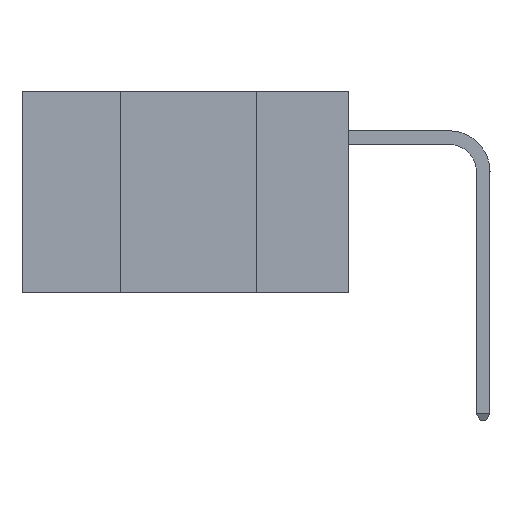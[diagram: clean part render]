
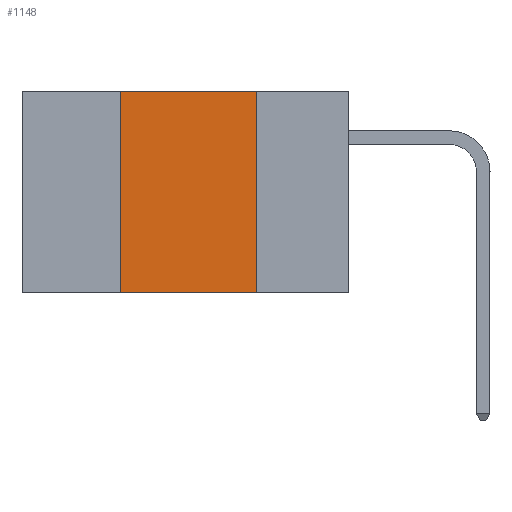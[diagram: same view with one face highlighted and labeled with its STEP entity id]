
A CAD part, left-side view. The second image highlights one B-rep face of the part: STEP entity #1148.
In plain terms, the highlighted planar face has unit normal (-1, 0, 0).
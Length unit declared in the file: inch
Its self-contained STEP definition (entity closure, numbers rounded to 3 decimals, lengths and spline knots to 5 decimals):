
#29 = EDGE_CURVE ( 'NONE', #10074, #1159, #582, .T. ) ;
#163 = VECTOR ( 'NONE', #11731, 39.37008 ) ;
#582 = LINE ( 'NONE', #8901, #915 ) ;
#915 = VECTOR ( 'NONE', #6069, 39.37008 ) ;
#1148 = ADVANCED_FACE ( 'NONE', ( #10179 ), #11896, .F. ) ;
#1159 = VERTEX_POINT ( 'NONE', #11498 ) ;
#2602 = VECTOR ( 'NONE', #3697, 39.37008 ) ;
#3254 = LINE ( 'NONE', #9978, #2602 ) ;
#3297 = DIRECTION ( 'NONE',  ( 0., 0., -1. ) ) ;
#3697 = DIRECTION ( 'NONE',  ( 0., -1., 0. ) ) ;
#4525 = CARTESIAN_POINT ( 'NONE',  ( 0., 0.42, 0. ) ) ;
#4973 = VECTOR ( 'NONE', #3297, 39.37008 ) ;
#5671 = EDGE_CURVE ( 'NONE', #12258, #6358, #3254, .T. ) ;
#5674 = LINE ( 'NONE', #4525, #163 ) ;
#6060 = ORIENTED_EDGE ( 'NONE', *, *, #11762, .F. ) ;
#6069 = DIRECTION ( 'NONE',  ( 0., -1., 0. ) ) ;
#6358 = VERTEX_POINT ( 'NONE', #9268 ) ;
#6430 = CARTESIAN_POINT ( 'NONE',  ( 0., 0.17, 0. ) ) ;
#6888 = CARTESIAN_POINT ( 'NONE',  ( 0., 0.42, 0. ) ) ;
#7001 = EDGE_CURVE ( 'NONE', #10074, #12258, #5674, .T. ) ;
#7787 = LINE ( 'NONE', #6430, #4973 ) ;
#8901 = CARTESIAN_POINT ( 'NONE',  ( 0., 0.6, -0.37 ) ) ;
#9268 = CARTESIAN_POINT ( 'NONE',  ( 0., 0.17, 0. ) ) ;
#9722 = CARTESIAN_POINT ( 'NONE',  ( 0., 0.42, -0.37 ) ) ;
#9978 = CARTESIAN_POINT ( 'NONE',  ( 0., 0.6, 0. ) ) ;
#10074 = VERTEX_POINT ( 'NONE', #9722 ) ;
#10179 = FACE_OUTER_BOUND ( 'NONE', #11513, .T. ) ;
#11498 = CARTESIAN_POINT ( 'NONE',  ( 0., 0.17, -0.37 ) ) ;
#11513 = EDGE_LOOP ( 'NONE', ( #6060, #12735, #13034, #12605 ) ) ;
#11731 = DIRECTION ( 'NONE',  ( 0., 0., 1. ) ) ;
#11745 = DIRECTION ( 'NONE',  ( 1., 0., 0. ) ) ;
#11762 = EDGE_CURVE ( 'NONE', #6358, #1159, #7787, .T. ) ;
#11808 = DIRECTION ( 'NONE',  ( 0., 0., -1. ) ) ;
#11839 = CARTESIAN_POINT ( 'NONE',  ( 0., 0.6, 0. ) ) ;
#11896 = PLANE ( 'NONE',  #13007 ) ;
#12258 = VERTEX_POINT ( 'NONE', #6888 ) ;
#12605 = ORIENTED_EDGE ( 'NONE', *, *, #29, .T. ) ;
#12735 = ORIENTED_EDGE ( 'NONE', *, *, #5671, .F. ) ;
#13007 = AXIS2_PLACEMENT_3D ( 'NONE', #11839, #11745, #11808 ) ;
#13034 = ORIENTED_EDGE ( 'NONE', *, *, #7001, .F. ) ;
